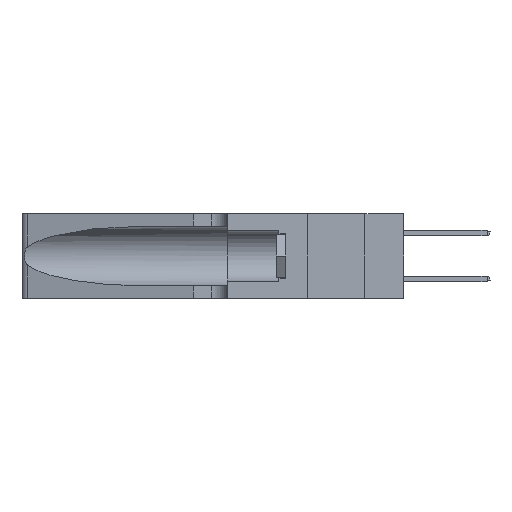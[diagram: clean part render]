
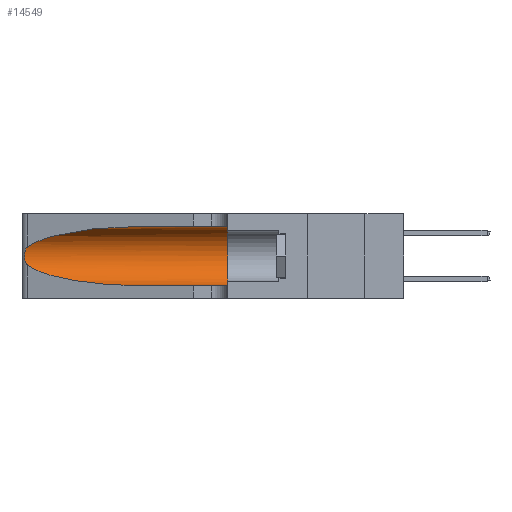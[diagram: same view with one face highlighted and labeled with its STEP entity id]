
A CAD part, left-side view. The second image highlights one B-rep face of the part: STEP entity #14549.
In plain terms, the highlighted cylindrical face has radius 3.308 mm (diameter 6.617 mm), a partial arc.
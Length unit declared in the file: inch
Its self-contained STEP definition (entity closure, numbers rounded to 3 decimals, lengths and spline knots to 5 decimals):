
#1020 = CARTESIAN_POINT ( 'NONE',  ( 0.1305, 0.72297, 0.05475 ) ) ;
#1260 = ORIENTED_EDGE ( 'NONE', *, *, #5220, .T. ) ;
#2087 = EDGE_CURVE ( 'NONE', #29222, #37317, #34823, .T. ) ;
#2328 = CARTESIAN_POINT ( 'NONE',  ( 0.26017, 1.23833, 0.17102 ) ) ;
#2716 = CARTESIAN_POINT ( 'NONE',  ( 0.25487, 1.22718, 0.22369 ) ) ;
#2957 = VERTEX_POINT ( 'NONE', #6112 ) ;
#5220 = EDGE_CURVE ( 'NONE', #37317, #22607, #28066, .T. ) ;
#5246 = CARTESIAN_POINT ( 'NONE',  ( 0.25789, 1.23486, 0.15765 ) ) ;
#5537 = CARTESIAN_POINT ( 'NONE',  ( 0.18966, 0.96281, 0.31525 ) ) ;
#6112 = CARTESIAN_POINT ( 'NONE',  ( 0.1305, 0.35, 0.05475 ) ) ;
#7176 = CARTESIAN_POINT ( 'NONE',  ( 0.1305, 0.35, 0.185 ) ) ;
#8066 = CARTESIAN_POINT ( 'NONE',  ( 0.25639, 1.23184, 0.21858 ) ) ;
#8186 = CARTESIAN_POINT ( 'NONE',  ( 0.25555, 1.22993, 0.14849 ) ) ;
#8412 = LINE ( 'NONE', #19898, #23175 ) ;
#9256 = CARTESIAN_POINT ( 'NONE',  ( 0.1305, 0.72297, 0.31525 ) ) ;
#9739 = CARTESIAN_POINT ( 'NONE',  ( 0.25487, 1.22718, 0.22369 ) ) ;
#10112 = DIRECTION ( 'NONE',  ( 0., 0., 1. ) ) ;
#10828 = ORIENTED_EDGE ( 'NONE', *, *, #21841, .T. ) ;
#11000 = DIRECTION ( 'NONE',  ( 0., -1., 0. ) ) ;
#11021 = CARTESIAN_POINT ( 'NONE',  ( 0.25487, 1.22718, 0.22369 ) ) ;
#12690 = CARTESIAN_POINT ( 'NONE',  ( 0.2373, 1.15595, 0.08982 ) ) ;
#14007 = CARTESIAN_POINT ( 'NONE',  ( 0.25787, 1.23484, 0.2124 ) ) ;
#14162 = ORIENTED_EDGE ( 'NONE', *, *, #31701, .F. ) ;
#14529 = FACE_OUTER_BOUND ( 'NONE', #15301, .T. ) ;
#14549 = ADVANCED_FACE ( 'NONE', ( #14529 ), #20526, .F. ) ;
#14972 = ORIENTED_EDGE ( 'NONE', *, *, #29304, .F. ) ;
#15301 = EDGE_LOOP ( 'NONE', ( #33662, #19113, #1260, #10828, #14972, #14162 ) ) ;
#15693 = CARTESIAN_POINT ( 'NONE',  ( 0.25487, 1.22718, 0.14631 ) ) ;
#16307 = VECTOR ( 'NONE', #17191, 39.37008 ) ;
#16961 = CARTESIAN_POINT ( 'NONE',  ( 0.1305, 1.61858, 0.185 ) ) ;
#16977 = CARTESIAN_POINT ( 'NONE',  ( 0.26018, 1.23835, 0.19895 ) ) ;
#17191 = DIRECTION ( 'NONE',  ( 0., -1., 0. ) ) ;
#18178 = VERTEX_POINT ( 'NONE', #9256 ) ;
#18417 =( BOUNDED_CURVE ( )  B_SPLINE_CURVE ( 3, ( #31960, #5537, #20350, #2716 ),
 .UNSPECIFIED., .F., .F. ) 
 B_SPLINE_CURVE_WITH_KNOTS ( ( 4, 4 ),
 ( 1.5708, 2.84003 ),
 .UNSPECIFIED. ) 
 CURVE ( )  GEOMETRIC_REPRESENTATION_ITEM ( )  RATIONAL_B_SPLINE_CURVE ( ( 1., 0.87, 0.87, 1. ) ) 
 REPRESENTATION_ITEM ( '' )  );
#18660 = CARTESIAN_POINT ( 'NONE',  ( 0.18966, 0.96281, 0.05475 ) ) ;
#18733 = CARTESIAN_POINT ( 'NONE',  ( 0.1305, 0.72297, 0.05475 ) ) ;
#19113 = ORIENTED_EDGE ( 'NONE', *, *, #2087, .T. ) ;
#19898 = CARTESIAN_POINT ( 'NONE',  ( 0.1305, 1.61858, 0.05475 ) ) ;
#19932 = CARTESIAN_POINT ( 'NONE',  ( 0.26075, 1.23896, 0.178 ) ) ;
#20130 = AXIS2_PLACEMENT_3D ( 'NONE', #16961, #11000, #31526 ) ;
#20350 = CARTESIAN_POINT ( 'NONE',  ( 0.2373, 1.15595, 0.28018 ) ) ;
#20526 = CYLINDRICAL_SURFACE ( 'NONE', #20130, 0.13025 ) ;
#21106 = CARTESIAN_POINT ( 'NONE',  ( 0.25487, 1.22718, 0.14631 ) ) ;
#21841 = EDGE_CURVE ( 'NONE', #22607, #2957, #8412, .T. ) ;
#22607 = VERTEX_POINT ( 'NONE', #18733 ) ;
#22852 = DIRECTION ( 'NONE',  ( 0., -1., 0. ) ) ;
#22888 = CARTESIAN_POINT ( 'NONE',  ( 0.25856, 1.23593, 0.16098 ) ) ;
#23175 = VECTOR ( 'NONE', #22852, 39.37008 ) ;
#23195 = LINE ( 'NONE', #37592, #16307 ) ;
#23408 = CARTESIAN_POINT ( 'NONE',  ( 0.1305, 0.35, 0.31525 ) ) ;
#25839 = CARTESIAN_POINT ( 'NONE',  ( 0.25639, 1.23186, 0.15144 ) ) ;
#27508 = VERTEX_POINT ( 'NONE', #23408 ) ;
#27748 = DIRECTION ( 'NONE',  ( 0., 1., 0. ) ) ;
#28066 =( BOUNDED_CURVE ( )  B_SPLINE_CURVE ( 3, ( #15693, #12690, #18660, #1020 ),
 .UNSPECIFIED., .F., .T. ) 
 B_SPLINE_CURVE_WITH_KNOTS ( ( 4, 4 ),
 ( 3.44316, 4.71239 ),
 .UNSPECIFIED. ) 
 CURVE ( )  GEOMETRIC_REPRESENTATION_ITEM ( )  RATIONAL_B_SPLINE_CURVE ( ( 1., 0.87, 0.87, 1. ) ) 
 REPRESENTATION_ITEM ( '' )  );
#28635 = CARTESIAN_POINT ( 'NONE',  ( 0.25555, 1.22994, 0.2215 ) ) ;
#28766 = CARTESIAN_POINT ( 'NONE',  ( 0.25487, 1.22718, 0.14631 ) ) ;
#28966 = EDGE_CURVE ( 'NONE', #18178, #29222, #18417, .T. ) ;
#29222 = VERTEX_POINT ( 'NONE', #9739 ) ;
#29304 = EDGE_CURVE ( 'NONE', #27508, #2957, #37054, .T. ) ;
#31526 = DIRECTION ( 'NONE',  ( 0., 0., -1. ) ) ;
#31701 = EDGE_CURVE ( 'NONE', #18178, #27508, #23195, .T. ) ;
#31960 = CARTESIAN_POINT ( 'NONE',  ( 0.1305, 0.72297, 0.31525 ) ) ;
#33662 = ORIENTED_EDGE ( 'NONE', *, *, #28966, .T. ) ;
#34282 = AXIS2_PLACEMENT_3D ( 'NONE', #7176, #27748, #10112 ) ;
#34484 = CARTESIAN_POINT ( 'NONE',  ( 0.25854, 1.2359, 0.20912 ) ) ;
#34823 = B_SPLINE_CURVE_WITH_KNOTS ( 'NONE', 3,
 ( #11021, #28635, #8066, #14007, #34484, #16977, #37380, #19932, #2328, #22888, #5246, #25839, #8186, #28766 ),
 .UNSPECIFIED., .F., .F.,
 ( 4, 2, 2, 2, 2, 2, 4 ),
 ( 0., 0.00027, 0.00053, 0.00107, 0.0016, 0.00187, 0.00214 ),
 .UNSPECIFIED. ) ;
#37054 = CIRCLE ( 'NONE', #34282, 0.13025 ) ;
#37317 = VERTEX_POINT ( 'NONE', #21106 ) ;
#37380 = CARTESIAN_POINT ( 'NONE',  ( 0.26075, 1.23896, 0.19203 ) ) ;
#37592 = CARTESIAN_POINT ( 'NONE',  ( 0.1305, 1.61858, 0.31525 ) ) ;
